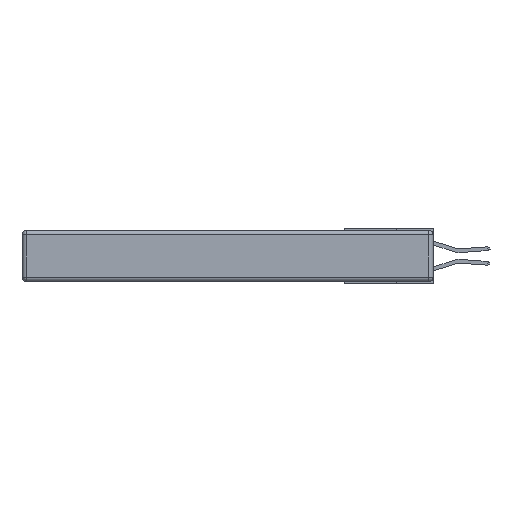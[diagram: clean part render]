
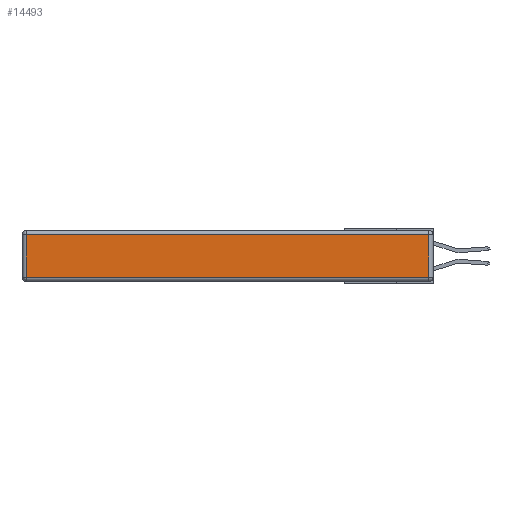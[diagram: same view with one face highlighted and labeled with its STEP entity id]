
A CAD part, left-side view. The second image highlights one B-rep face of the part: STEP entity #14493.
In plain terms, the highlighted planar face has unit normal (-1, 0, 0).
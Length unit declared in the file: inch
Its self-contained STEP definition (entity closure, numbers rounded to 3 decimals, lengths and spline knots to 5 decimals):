
#1426 = CARTESIAN_POINT ( 'NONE',  ( 0., 0.03, -0.343 ) ) ;
#3473 = DIRECTION ( 'NONE',  ( 0., 1., 0. ) ) ;
#3579 = LINE ( 'NONE', #34485, #22766 ) ;
#3735 = EDGE_CURVE ( 'NONE', #30405, #17058, #32189, .T. ) ;
#6596 = DIRECTION ( 'NONE',  ( 0., 0., -1. ) ) ;
#7513 = AXIS2_PLACEMENT_3D ( 'NONE', #21230, #18779, #35425 ) ;
#7805 = VECTOR ( 'NONE', #3473, 39.37008 ) ;
#8688 = EDGE_CURVE ( 'NONE', #24457, #30405, #28762, .T. ) ;
#8820 = VECTOR ( 'NONE', #6596, 39.37008 ) ;
#10362 = FACE_OUTER_BOUND ( 'NONE', #27320, .T. ) ;
#10926 = ORIENTED_EDGE ( 'NONE', *, *, #3735, .T. ) ;
#12161 = CARTESIAN_POINT ( 'NONE',  ( 0., 0.03, -0.313 ) ) ;
#14493 = ADVANCED_FACE ( 'NONE', ( #10362 ), #26922, .T. ) ;
#14912 = DIRECTION ( 'NONE',  ( 0., -1., 0. ) ) ;
#17058 = VERTEX_POINT ( 'NONE', #23085 ) ;
#17730 = ORIENTED_EDGE ( 'NONE', *, *, #26140, .T. ) ;
#18779 = DIRECTION ( 'NONE',  ( -1., 0., 0. ) ) ;
#19784 = ORIENTED_EDGE ( 'NONE', *, *, #26536, .T. ) ;
#21230 = CARTESIAN_POINT ( 'NONE',  ( 0., 0., -0.343 ) ) ;
#22487 = VERTEX_POINT ( 'NONE', #33941 ) ;
#22766 = VECTOR ( 'NONE', #14912, 39.37008 ) ;
#23085 = CARTESIAN_POINT ( 'NONE',  ( 0., 2.72, -0.03 ) ) ;
#23598 = LINE ( 'NONE', #26295, #8820 ) ;
#24457 = VERTEX_POINT ( 'NONE', #12161 ) ;
#26140 = EDGE_CURVE ( 'NONE', #22487, #24457, #3579, .T. ) ;
#26295 = CARTESIAN_POINT ( 'NONE',  ( 0., 2.72, -0.343 ) ) ;
#26536 = EDGE_CURVE ( 'NONE', #17058, #22487, #23598, .T. ) ;
#26922 = PLANE ( 'NONE',  #7513 ) ;
#27320 = EDGE_LOOP ( 'NONE', ( #17730, #31996, #10926, #19784 ) ) ;
#27492 = VECTOR ( 'NONE', #31965, 39.37008 ) ;
#28762 = LINE ( 'NONE', #1426, #27492 ) ;
#30405 = VERTEX_POINT ( 'NONE', #30707 ) ;
#30707 = CARTESIAN_POINT ( 'NONE',  ( 0., 0.03, -0.03 ) ) ;
#31309 = CARTESIAN_POINT ( 'NONE',  ( 0., 2.75, -0.03 ) ) ;
#31965 = DIRECTION ( 'NONE',  ( 0., 0., 1. ) ) ;
#31996 = ORIENTED_EDGE ( 'NONE', *, *, #8688, .T. ) ;
#32189 = LINE ( 'NONE', #31309, #7805 ) ;
#33941 = CARTESIAN_POINT ( 'NONE',  ( 0., 2.72, -0.313 ) ) ;
#34485 = CARTESIAN_POINT ( 'NONE',  ( 0., 0., -0.313 ) ) ;
#35425 = DIRECTION ( 'NONE',  ( 0., 0., 1. ) ) ;
